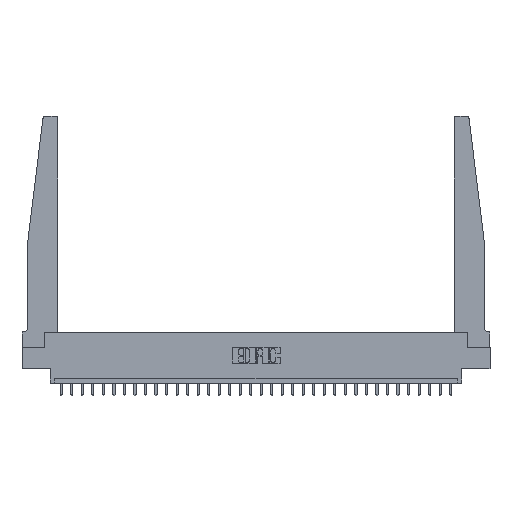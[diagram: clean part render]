
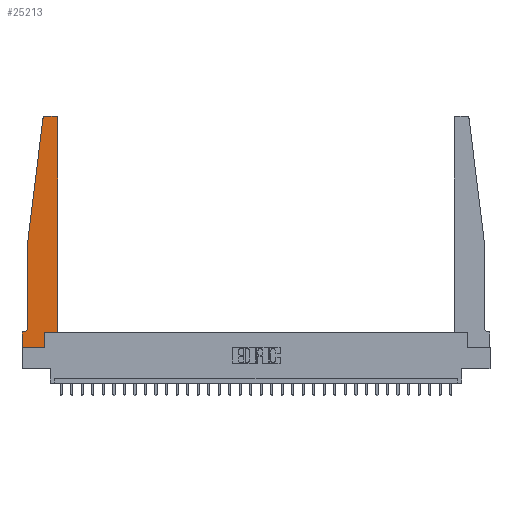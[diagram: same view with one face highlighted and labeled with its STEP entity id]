
A CAD part, top view. The second image highlights one B-rep face of the part: STEP entity #25213.
In plain terms, the highlighted planar face has unit normal (0, 0, 1).
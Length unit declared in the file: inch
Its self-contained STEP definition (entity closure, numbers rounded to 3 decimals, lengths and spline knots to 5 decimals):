
#55 = EDGE_CURVE ( 'NONE', #12714, #3790, #16335, .T. ) ;
#952 = VECTOR ( 'NONE', #2589, 39.37008 ) ;
#1375 = CARTESIAN_POINT ( 'NONE',  ( 0.2605, 0.18, 0.37 ) ) ;
#1645 = DIRECTION ( 'NONE',  ( 1., 0., 0. ) ) ;
#1763 = AXIS2_PLACEMENT_3D ( 'NONE', #4031, #5963, #1645 ) ;
#2152 = CARTESIAN_POINT ( 'NONE',  ( 0.015, 0.1875, 0.37 ) ) ;
#2194 = CARTESIAN_POINT ( 'NONE',  ( 0., 0.1875, 0.37 ) ) ;
#2269 = EDGE_LOOP ( 'NONE', ( #28291, #5876, #5033, #18917, #4607, #10048, #28484, #10028, #6275, #25378, #18702, #13776 ) ) ;
#2589 = DIRECTION ( 'NONE',  ( -0.122, -0.992, 0. ) ) ;
#2763 = CARTESIAN_POINT ( 'NONE',  ( 0.25, 2.75, 0.37 ) ) ;
#3083 = EDGE_CURVE ( 'NONE', #3790, #17080, #23035, .T. ) ;
#3157 = EDGE_CURVE ( 'NONE', #12488, #28961, #16846, .T. ) ;
#3608 = EDGE_CURVE ( 'NONE', #17611, #11573, #26383, .T. ) ;
#3790 = VERTEX_POINT ( 'NONE', #13207 ) ;
#4031 = CARTESIAN_POINT ( 'NONE',  ( 0., 0.1875, 0.37 ) ) ;
#4073 = CARTESIAN_POINT ( 'NONE',  ( 0.2605, 0.18, 0.37 ) ) ;
#4188 = EDGE_CURVE ( 'NONE', #21468, #17611, #16979, .T. ) ;
#4318 = VECTOR ( 'NONE', #14885, 39.37008 ) ;
#4607 = ORIENTED_EDGE ( 'NONE', *, *, #3608, .T. ) ;
#5033 = ORIENTED_EDGE ( 'NONE', *, *, #19844, .T. ) ;
#5275 = VECTOR ( 'NONE', #18144, 39.37008 ) ;
#5876 = ORIENTED_EDGE ( 'NONE', *, *, #3083, .T. ) ;
#5952 = EDGE_CURVE ( 'NONE', #20156, #12714, #14614, .T. ) ;
#5963 = DIRECTION ( 'NONE',  ( 0., 0., 1. ) ) ;
#6149 = DIRECTION ( 'NONE',  ( 0., 1., 0. ) ) ;
#6275 = ORIENTED_EDGE ( 'NONE', *, *, #22242, .T. ) ;
#6765 = VERTEX_POINT ( 'NONE', #4073 ) ;
#7120 = LINE ( 'NONE', #16186, #13791 ) ;
#7361 = VECTOR ( 'NONE', #21773, 39.37008 ) ;
#7672 = CARTESIAN_POINT ( 'NONE',  ( 0.065, 1.25, 0.37 ) ) ;
#8040 = CARTESIAN_POINT ( 'NONE',  ( 0.425, 0.18, 0.37 ) ) ;
#8332 = DIRECTION ( 'NONE',  ( 1., 0., 0. ) ) ;
#8369 = EDGE_CURVE ( 'NONE', #28961, #26976, #19512, .T. ) ;
#10028 = ORIENTED_EDGE ( 'NONE', *, *, #8369, .T. ) ;
#10048 = ORIENTED_EDGE ( 'NONE', *, *, #22516, .T. ) ;
#10163 = AXIS2_PLACEMENT_3D ( 'NONE', #27775, #23443, #20742 ) ;
#10234 = VECTOR ( 'NONE', #6149, 39.37008 ) ;
#10372 = DIRECTION ( 'NONE',  ( 0., 0., -1. ) ) ;
#10513 = CARTESIAN_POINT ( 'NONE',  ( 0.24675, 2.72367, 0.37 ) ) ;
#11248 = DIRECTION ( 'NONE',  ( 0., 0., 1. ) ) ;
#11573 = VERTEX_POINT ( 'NONE', #2152 ) ;
#11639 = AXIS2_PLACEMENT_3D ( 'NONE', #24548, #10372, #29169 ) ;
#11762 = EDGE_CURVE ( 'NONE', #6765, #17650, #7120, .T. ) ;
#11957 = CARTESIAN_POINT ( 'NONE',  ( 0.065, 0.1875, 0.37 ) ) ;
#12111 = DIRECTION ( 'NONE',  ( 0., -1., 0. ) ) ;
#12155 = LINE ( 'NONE', #7672, #952 ) ;
#12201 = VECTOR ( 'NONE', #25500, 39.37008 ) ;
#12488 = VERTEX_POINT ( 'NONE', #2194 ) ;
#12714 = VERTEX_POINT ( 'NONE', #16789 ) ;
#13207 = CARTESIAN_POINT ( 'NONE',  ( 0.27653, 2.75, 0.37 ) ) ;
#13776 = ORIENTED_EDGE ( 'NONE', *, *, #5952, .T. ) ;
#13791 = VECTOR ( 'NONE', #25296, 39.37008 ) ;
#14482 = CARTESIAN_POINT ( 'NONE',  ( 0., 0., 0.37 ) ) ;
#14614 = CIRCLE ( 'NONE', #19877, 0.03 ) ;
#14885 = DIRECTION ( 'NONE',  ( 0., 1., 0. ) ) ;
#16186 = CARTESIAN_POINT ( 'NONE',  ( 0.425, 0.18, 0.37 ) ) ;
#16335 = LINE ( 'NONE', #2763, #5275 ) ;
#16789 = CARTESIAN_POINT ( 'NONE',  ( 0.395, 2.75, 0.37 ) ) ;
#16846 = LINE ( 'NONE', #14482, #7361 ) ;
#16979 = LINE ( 'NONE', #21181, #19747 ) ;
#17080 = VERTEX_POINT ( 'NONE', #10513 ) ;
#17086 = CARTESIAN_POINT ( 'NONE',  ( 0.395, 2.72, 0.37 ) ) ;
#17258 = LINE ( 'NONE', #8040, #4318 ) ;
#17610 = LINE ( 'NONE', #1375, #10234 ) ;
#17611 = VERTEX_POINT ( 'NONE', #22068 ) ;
#17650 = VERTEX_POINT ( 'NONE', #29086 ) ;
#18087 = DIRECTION ( 'NONE',  ( 1., 0., 0. ) ) ;
#18144 = DIRECTION ( 'NONE',  ( -1., 0., 0. ) ) ;
#18257 = CARTESIAN_POINT ( 'NONE',  ( 0.2605, 0., 0.37 ) ) ;
#18702 = ORIENTED_EDGE ( 'NONE', *, *, #20812, .T. ) ;
#18917 = ORIENTED_EDGE ( 'NONE', *, *, #4188, .T. ) ;
#19512 = LINE ( 'NONE', #24595, #27100 ) ;
#19747 = VECTOR ( 'NONE', #12111, 39.37008 ) ;
#19833 = CARTESIAN_POINT ( 'NONE',  ( 0., 0., 0.37 ) ) ;
#19844 = EDGE_CURVE ( 'NONE', #17080, #21468, #12155, .T. ) ;
#19877 = AXIS2_PLACEMENT_3D ( 'NONE', #17086, #11248, #18087 ) ;
#20156 = VERTEX_POINT ( 'NONE', #24368 ) ;
#20742 = DIRECTION ( 'NONE',  ( 1., 0., 0. ) ) ;
#20812 = EDGE_CURVE ( 'NONE', #17650, #20156, #17258, .T. ) ;
#21181 = CARTESIAN_POINT ( 'NONE',  ( 0.065, 1.25, 0.37 ) ) ;
#21468 = VERTEX_POINT ( 'NONE', #25768 ) ;
#21773 = DIRECTION ( 'NONE',  ( 0., -1., 0. ) ) ;
#22068 = CARTESIAN_POINT ( 'NONE',  ( 0.065, 0.2375, 0.37 ) ) ;
#22242 = EDGE_CURVE ( 'NONE', #26976, #6765, #17610, .T. ) ;
#22516 = EDGE_CURVE ( 'NONE', #11573, #12488, #23960, .T. ) ;
#23035 = CIRCLE ( 'NONE', #10163, 0.03 ) ;
#23443 = DIRECTION ( 'NONE',  ( 0., 0., 1. ) ) ;
#23960 = LINE ( 'NONE', #11957, #12201 ) ;
#24368 = CARTESIAN_POINT ( 'NONE',  ( 0.425, 2.72, 0.37 ) ) ;
#24461 = PLANE ( 'NONE',  #1763 ) ;
#24548 = CARTESIAN_POINT ( 'NONE',  ( 0.015, 0.2375, 0.37 ) ) ;
#24595 = CARTESIAN_POINT ( 'NONE',  ( 0., 0., 0.37 ) ) ;
#25213 = ADVANCED_FACE ( 'NONE', ( #26561 ), #24461, .T. ) ;
#25296 = DIRECTION ( 'NONE',  ( 1., 0., 0. ) ) ;
#25378 = ORIENTED_EDGE ( 'NONE', *, *, #11762, .T. ) ;
#25500 = DIRECTION ( 'NONE',  ( -1., 0., 0. ) ) ;
#25768 = CARTESIAN_POINT ( 'NONE',  ( 0.065, 1.25, 0.37 ) ) ;
#26383 = CIRCLE ( 'NONE', #11639, 0.05 ) ;
#26561 = FACE_OUTER_BOUND ( 'NONE', #2269, .T. ) ;
#26976 = VERTEX_POINT ( 'NONE', #18257 ) ;
#27100 = VECTOR ( 'NONE', #8332, 39.37008 ) ;
#27775 = CARTESIAN_POINT ( 'NONE',  ( 0.27653, 2.72, 0.37 ) ) ;
#28291 = ORIENTED_EDGE ( 'NONE', *, *, #55, .T. ) ;
#28484 = ORIENTED_EDGE ( 'NONE', *, *, #3157, .T. ) ;
#28961 = VERTEX_POINT ( 'NONE', #19833 ) ;
#29086 = CARTESIAN_POINT ( 'NONE',  ( 0.425, 0.18, 0.37 ) ) ;
#29169 = DIRECTION ( 'NONE',  ( -1., 0., 0. ) ) ;
